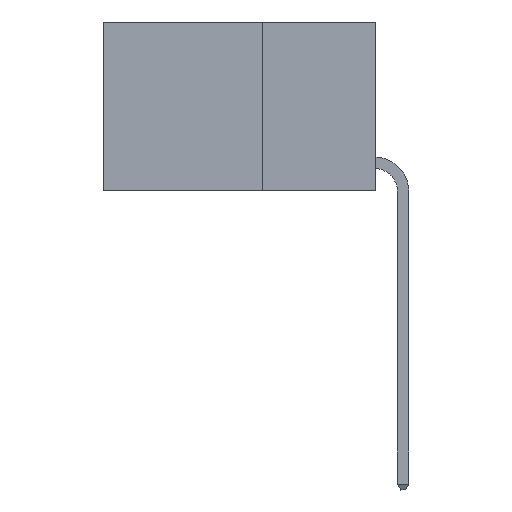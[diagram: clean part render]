
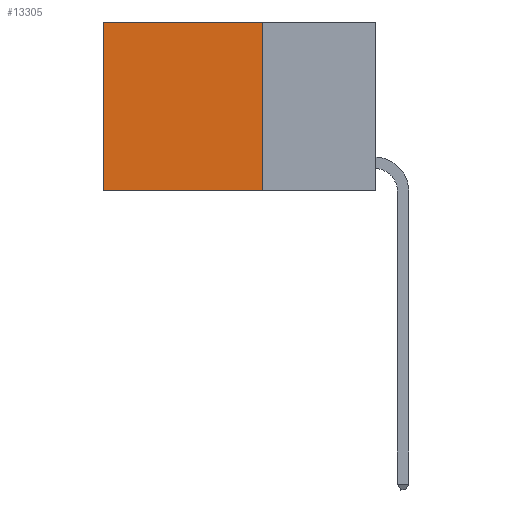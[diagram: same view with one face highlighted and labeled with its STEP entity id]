
A CAD part, left-side view. The second image highlights one B-rep face of the part: STEP entity #13305.
In plain terms, the highlighted planar face has unit normal (-1, 0, 0).
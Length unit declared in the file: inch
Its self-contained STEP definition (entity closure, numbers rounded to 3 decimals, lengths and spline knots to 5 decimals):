
#203 = VECTOR ( 'NONE', #4314, 39.37008 ) ;
#243 = CARTESIAN_POINT ( 'NONE',  ( 0.2625, 0.25, 0. ) ) ;
#2276 = LINE ( 'NONE', #10018, #20064 ) ;
#3102 = DIRECTION ( 'NONE',  ( 0., 0., -1. ) ) ;
#4314 = DIRECTION ( 'NONE',  ( 0., 1., 0. ) ) ;
#6094 = DIRECTION ( 'NONE',  ( 0., 0., -1. ) ) ;
#7434 = VERTEX_POINT ( 'NONE', #21841 ) ;
#9129 = LINE ( 'NONE', #11179, #12418 ) ;
#9139 = VERTEX_POINT ( 'NONE', #15991 ) ;
#10018 = CARTESIAN_POINT ( 'NONE',  ( 0.2625, 0.6, 0. ) ) ;
#10162 = CARTESIAN_POINT ( 'NONE',  ( 0.2625, 0.25, 0. ) ) ;
#10439 = EDGE_LOOP ( 'NONE', ( #15475, #20608, #12355, #11597 ) ) ;
#11179 = CARTESIAN_POINT ( 'NONE',  ( 0.2625, 0.25, -0.37 ) ) ;
#11597 = ORIENTED_EDGE ( 'NONE', *, *, #13294, .T. ) ;
#11985 = AXIS2_PLACEMENT_3D ( 'NONE', #10162, #17917, #19474 ) ;
#12355 = ORIENTED_EDGE ( 'NONE', *, *, #14534, .F. ) ;
#12418 = VECTOR ( 'NONE', #22616, 39.37008 ) ;
#12464 = VERTEX_POINT ( 'NONE', #17758 ) ;
#12991 = LINE ( 'NONE', #18989, #16904 ) ;
#13294 = EDGE_CURVE ( 'NONE', #22471, #12464, #13588, .T. ) ;
#13305 = ADVANCED_FACE ( 'NONE', ( #13836 ), #21619, .F. ) ;
#13585 = EDGE_CURVE ( 'NONE', #7434, #9139, #9129, .T. ) ;
#13588 = LINE ( 'NONE', #243, #203 ) ;
#13836 = FACE_OUTER_BOUND ( 'NONE', #10439, .T. ) ;
#14534 = EDGE_CURVE ( 'NONE', #22471, #7434, #12991, .T. ) ;
#15475 = ORIENTED_EDGE ( 'NONE', *, *, #24025, .T. ) ;
#15991 = CARTESIAN_POINT ( 'NONE',  ( 0.2625, 0.6, -0.37 ) ) ;
#16904 = VECTOR ( 'NONE', #3102, 39.37008 ) ;
#17758 = CARTESIAN_POINT ( 'NONE',  ( 0.2625, 0.6, 0. ) ) ;
#17917 = DIRECTION ( 'NONE',  ( 1., 0., 0. ) ) ;
#18989 = CARTESIAN_POINT ( 'NONE',  ( 0.2625, 0.25, 0. ) ) ;
#19474 = DIRECTION ( 'NONE',  ( 0., 0., -1. ) ) ;
#20064 = VECTOR ( 'NONE', #6094, 39.37008 ) ;
#20608 = ORIENTED_EDGE ( 'NONE', *, *, #13585, .F. ) ;
#21619 = PLANE ( 'NONE',  #11985 ) ;
#21841 = CARTESIAN_POINT ( 'NONE',  ( 0.2625, 0.25, -0.37 ) ) ;
#22471 = VERTEX_POINT ( 'NONE', #23179 ) ;
#22616 = DIRECTION ( 'NONE',  ( 0., 1., 0. ) ) ;
#23179 = CARTESIAN_POINT ( 'NONE',  ( 0.2625, 0.25, 0. ) ) ;
#24025 = EDGE_CURVE ( 'NONE', #12464, #9139, #2276, .T. ) ;
